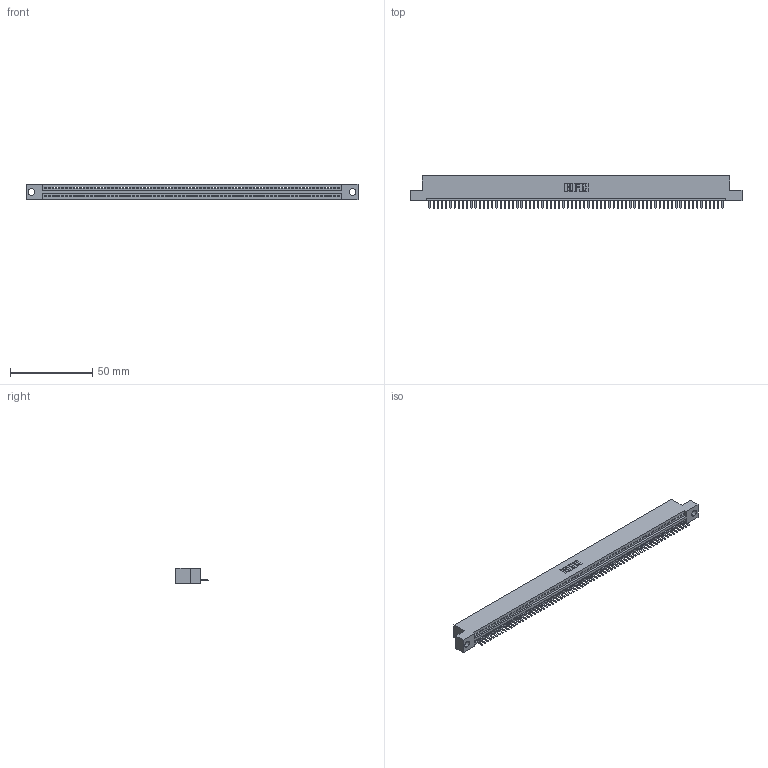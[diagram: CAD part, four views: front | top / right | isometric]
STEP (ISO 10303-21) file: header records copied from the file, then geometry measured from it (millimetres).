
FILE_DESCRIPTION (( 'STEP AP203' ), '1' );
FILE_NAME ('345-071-520-104.STEP', '2018-10-01T12:35:02', ( '' ), ( '' ), 'SwSTEP 2.0', 'SolidWorks 2016', '' );
FILE_SCHEMA (( 'CONFIG_CONTROL_DESIGN' ));
Length unit declared in the file: inch
Products named in the file (3): 345-071-520-104; 345-292-001_345-293-120; 345 Part_Flush Mounting Lugs - 0.156 Dia-TH
Assembly tree (72 placements, depth 2):
  345-071-520-104
    345 Part_Flush Mounting Lugs - 0.156 Dia-TH
    345-292-001_345-293-120  x71
Bounding box: 201.55 x 19.68 x 9.4 mm (x, y, z)
Volume: 19088.8 mm3; surface area: 24902 mm2
Topology: 72 solids, 72 shells, 4528 faces, 13405 edges, 8746 vertices
Faces by surface type: plane 3062, cylinder 1466
Entity records: 49649 total; most frequent: CARTESIAN_POINT 8617, ORIENTED_EDGE 8610, DIRECTION 7471, EDGE_CURVE 4305, LINE 3885, VECTOR 3885, VERTEX_POINT 2866, AXIS2_PLACEMENT_3D 1793
